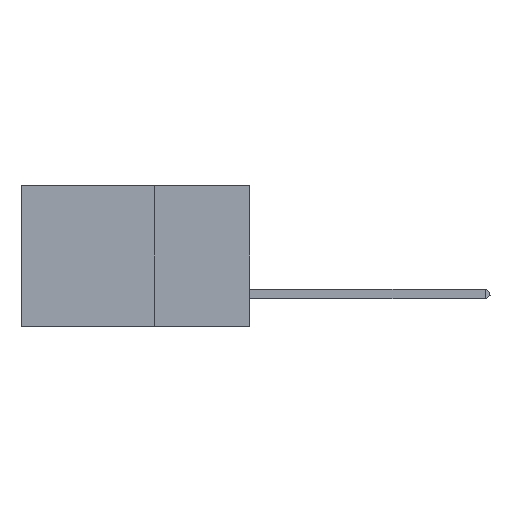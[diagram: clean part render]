
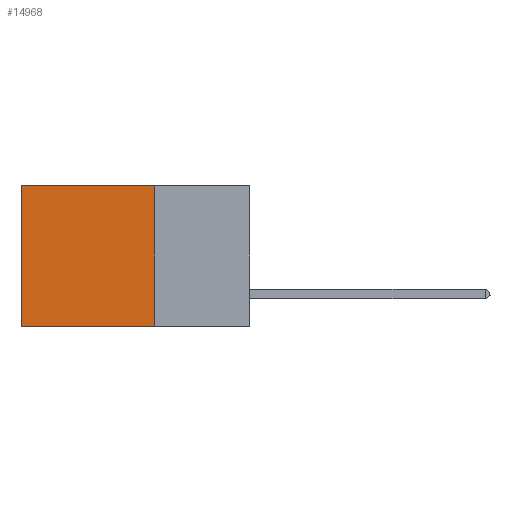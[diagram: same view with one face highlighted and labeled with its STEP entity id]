
A CAD part, left-side view. The second image highlights one B-rep face of the part: STEP entity #14968.
In plain terms, the highlighted planar face has unit normal (-1, 0, 0).
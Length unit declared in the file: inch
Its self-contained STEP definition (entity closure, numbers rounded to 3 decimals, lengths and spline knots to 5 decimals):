
#163 = PLANE ( 'NONE',  #15220 ) ;
#327 = CARTESIAN_POINT ( 'NONE',  ( 0.2875, 0.6, 0. ) ) ;
#899 = VERTEX_POINT ( 'NONE', #10178 ) ;
#1547 = LINE ( 'NONE', #327, #13188 ) ;
#1681 = DIRECTION ( 'NONE',  ( 1., 0., 0. ) ) ;
#2191 = DIRECTION ( 'NONE',  ( 0., 0., -1. ) ) ;
#2757 = ORIENTED_EDGE ( 'NONE', *, *, #7349, .T. ) ;
#4835 = DIRECTION ( 'NONE',  ( 0., 0., -1. ) ) ;
#5028 = CARTESIAN_POINT ( 'NONE',  ( 0.2875, 0.25, -0.37 ) ) ;
#6541 = CARTESIAN_POINT ( 'NONE',  ( 0.2875, 0.25, 0. ) ) ;
#6736 = DIRECTION ( 'NONE',  ( 0., 1., 0. ) ) ;
#6870 = CARTESIAN_POINT ( 'NONE',  ( 0.2875, 0.6, 0. ) ) ;
#7285 = VECTOR ( 'NONE', #6736, 39.37008 ) ;
#7349 = EDGE_CURVE ( 'NONE', #9234, #8398, #1547, .T. ) ;
#8102 = CARTESIAN_POINT ( 'NONE',  ( 0.2875, 0.25, -0.37 ) ) ;
#8398 = VERTEX_POINT ( 'NONE', #10566 ) ;
#8459 = VERTEX_POINT ( 'NONE', #5028 ) ;
#8478 = LINE ( 'NONE', #6541, #7285 ) ;
#8709 = VECTOR ( 'NONE', #11101, 39.37008 ) ;
#9234 = VERTEX_POINT ( 'NONE', #6870 ) ;
#9494 = DIRECTION ( 'NONE',  ( 0., 0., -1. ) ) ;
#9820 = CARTESIAN_POINT ( 'NONE',  ( 0.2875, 0.25, 0. ) ) ;
#10178 = CARTESIAN_POINT ( 'NONE',  ( 0.2875, 0.25, 0. ) ) ;
#10208 = ORIENTED_EDGE ( 'NONE', *, *, #11964, .F. ) ;
#10566 = CARTESIAN_POINT ( 'NONE',  ( 0.2875, 0.6, -0.37 ) ) ;
#11101 = DIRECTION ( 'NONE',  ( 0., 1., 0. ) ) ;
#11204 = ORIENTED_EDGE ( 'NONE', *, *, #11953, .F. ) ;
#11953 = EDGE_CURVE ( 'NONE', #899, #8459, #15744, .T. ) ;
#11964 = EDGE_CURVE ( 'NONE', #8459, #8398, #18051, .T. ) ;
#12285 = EDGE_CURVE ( 'NONE', #899, #9234, #8478, .T. ) ;
#12313 = CARTESIAN_POINT ( 'NONE',  ( 0.2875, 0.25, 0. ) ) ;
#12471 = ORIENTED_EDGE ( 'NONE', *, *, #12285, .T. ) ;
#12676 = VECTOR ( 'NONE', #2191, 39.37008 ) ;
#13188 = VECTOR ( 'NONE', #9494, 39.37008 ) ;
#14628 = FACE_OUTER_BOUND ( 'NONE', #15535, .T. ) ;
#14968 = ADVANCED_FACE ( 'NONE', ( #14628 ), #163, .F. ) ;
#15220 = AXIS2_PLACEMENT_3D ( 'NONE', #12313, #1681, #4835 ) ;
#15535 = EDGE_LOOP ( 'NONE', ( #2757, #10208, #11204, #12471 ) ) ;
#15744 = LINE ( 'NONE', #9820, #12676 ) ;
#18051 = LINE ( 'NONE', #8102, #8709 ) ;
